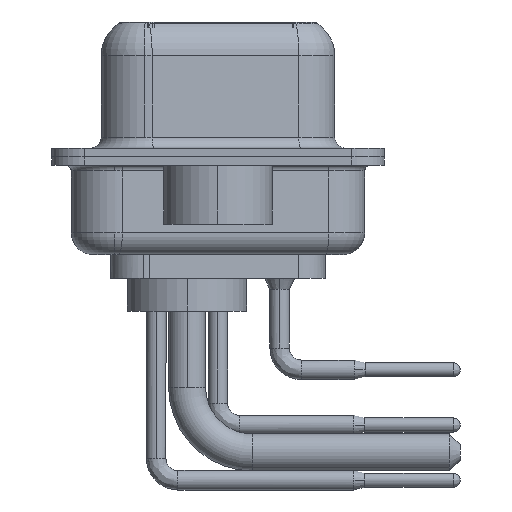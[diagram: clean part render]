
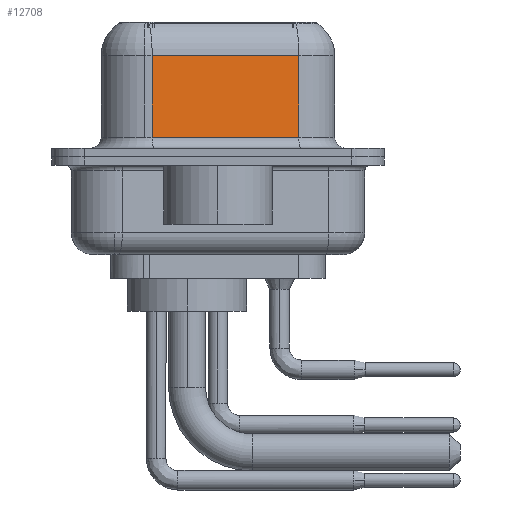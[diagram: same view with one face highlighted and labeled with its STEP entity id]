
A CAD part, left-side view. The second image highlights one B-rep face of the part: STEP entity #12708.
In plain terms, the highlighted planar face has unit normal (-0.985, -0.174, 0).
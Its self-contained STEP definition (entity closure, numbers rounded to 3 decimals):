
#2711 = DIRECTION ( 'NONE',  ( 0.174, -0.985, 0. ) ) ;
#2942 = CARTESIAN_POINT ( 'NONE',  ( 5.621, -3.722, 4.65 ) ) ;
#3901 = EDGE_CURVE ( 'NONE', #23814, #8998, #19141, .T. ) ;
#4276 = CARTESIAN_POINT ( 'NONE',  ( 5.621, -3.722, 4.65 ) ) ;
#5424 = DIRECTION ( 'NONE',  ( -0.174, 0.985, 0. ) ) ;
#6178 = EDGE_CURVE ( 'NONE', #6952, #8998, #8148, .T. ) ;
#6952 = VERTEX_POINT ( 'NONE', #26730 ) ;
#6960 = LINE ( 'NONE', #2942, #21707 ) ;
#7019 = ORIENTED_EDGE ( 'NONE', *, *, #15063, .T. ) ;
#7021 = PLANE ( 'NONE',  #16656 ) ;
#7031 = ORIENTED_EDGE ( 'NONE', *, *, #3901, .F. ) ;
#7658 = CARTESIAN_POINT ( 'NONE',  ( 5.621, -3.722, 0.9 ) ) ;
#7791 = VECTOR ( 'NONE', #9418, 1000. ) ;
#8148 = LINE ( 'NONE', #7658, #30571 ) ;
#8998 = VERTEX_POINT ( 'NONE', #28494 ) ;
#9418 = DIRECTION ( 'NONE',  ( 0., 0., -1. ) ) ;
#9781 = LINE ( 'NONE', #19833, #21420 ) ;
#12131 = CARTESIAN_POINT ( 'NONE',  ( 5.621, -3.722, 6.4 ) ) ;
#12452 = DIRECTION ( 'NONE',  ( 0.985, 0.174, 0. ) ) ;
#12708 = ADVANCED_FACE ( 'NONE', ( #29768 ), #7021, .F. ) ;
#13869 = CARTESIAN_POINT ( 'NONE',  ( 5.621, -3.722, 6.4 ) ) ;
#15063 = EDGE_CURVE ( 'NONE', #23814, #17153, #6960, .T. ) ;
#15092 = DIRECTION ( 'NONE',  ( -0.174, 0.985, 0. ) ) ;
#15515 = CARTESIAN_POINT ( 'NONE',  ( 4.43, 3.028, 4.65 ) ) ;
#16656 = AXIS2_PLACEMENT_3D ( 'NONE', #12131, #12452, #15092 ) ;
#17153 = VERTEX_POINT ( 'NONE', #15515 ) ;
#19141 = LINE ( 'NONE', #13869, #7791 ) ;
#19207 = EDGE_LOOP ( 'NONE', ( #7031, #7019, #24312, #22147 ) ) ;
#19833 = CARTESIAN_POINT ( 'NONE',  ( 4.43, 3.028, 6.4 ) ) ;
#20525 = EDGE_CURVE ( 'NONE', #17153, #6952, #9781, .T. ) ;
#21420 = VECTOR ( 'NONE', #29889, 1000. ) ;
#21707 = VECTOR ( 'NONE', #5424, 1000. ) ;
#22147 = ORIENTED_EDGE ( 'NONE', *, *, #6178, .T. ) ;
#23814 = VERTEX_POINT ( 'NONE', #4276 ) ;
#24312 = ORIENTED_EDGE ( 'NONE', *, *, #20525, .T. ) ;
#26730 = CARTESIAN_POINT ( 'NONE',  ( 4.43, 3.028, 0.9 ) ) ;
#28494 = CARTESIAN_POINT ( 'NONE',  ( 5.621, -3.722, 0.9 ) ) ;
#29768 = FACE_OUTER_BOUND ( 'NONE', #19207, .T. ) ;
#29889 = DIRECTION ( 'NONE',  ( 0., 0., -1. ) ) ;
#30571 = VECTOR ( 'NONE', #2711, 1000. ) ;
